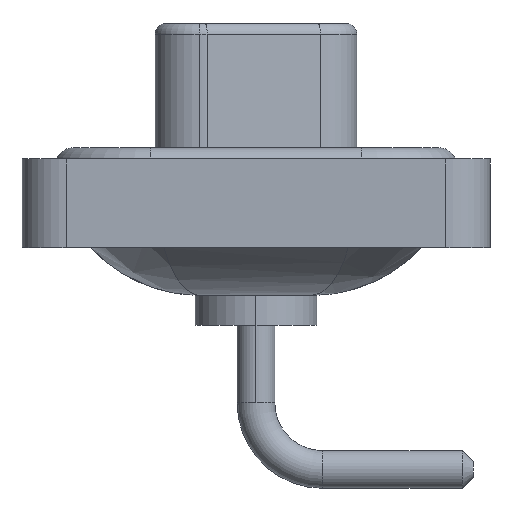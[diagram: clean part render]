
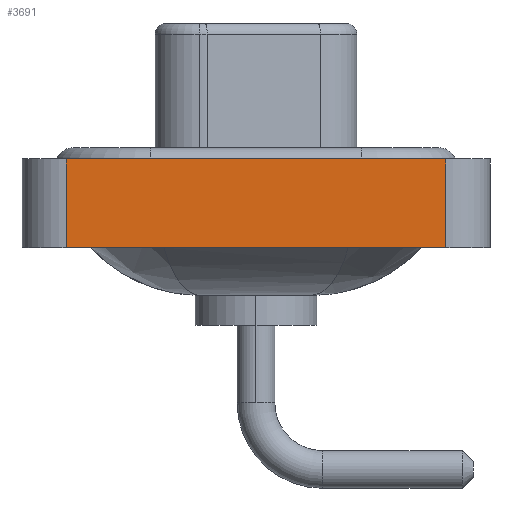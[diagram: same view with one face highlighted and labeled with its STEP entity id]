
A CAD part, left-side view. The second image highlights one B-rep face of the part: STEP entity #3691.
In plain terms, the highlighted planar face has unit normal (-1, 0, 0).
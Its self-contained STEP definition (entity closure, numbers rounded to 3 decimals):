
#387 = EDGE_CURVE ( 'NONE', #12388, #12974, #7501, .T. ) ;
#669 = VERTEX_POINT ( 'NONE', #12848 ) ;
#1430 = ORIENTED_EDGE ( 'NONE', *, *, #1746, .F. ) ;
#1504 = VECTOR ( 'NONE', #5171, 1000. ) ;
#1746 = EDGE_CURVE ( 'NONE', #12974, #669, #2811, .T. ) ;
#2571 = CARTESIAN_POINT ( 'NONE',  ( -7.25, -8.55, -3.6 ) ) ;
#2750 = EDGE_CURVE ( 'NONE', #5761, #669, #7914, .T. ) ;
#2811 = LINE ( 'NONE', #14663, #1504 ) ;
#3085 = LINE ( 'NONE', #9753, #5399 ) ;
#3217 = ORIENTED_EDGE ( 'NONE', *, *, #2750, .T. ) ;
#3414 = PLANE ( 'NONE',  #12436 ) ;
#3490 = DIRECTION ( 'NONE',  ( -1., 0., 0. ) ) ;
#3691 = ADVANCED_FACE ( 'NONE', ( #12682 ), #3414, .T. ) ;
#3801 = EDGE_CURVE ( 'NONE', #12388, #5761, #3085, .T. ) ;
#4676 = ORIENTED_EDGE ( 'NONE', *, *, #387, .F. ) ;
#5171 = DIRECTION ( 'NONE',  ( 0., -1., 0. ) ) ;
#5399 = VECTOR ( 'NONE', #8614, 1000. ) ;
#5761 = VERTEX_POINT ( 'NONE', #2571 ) ;
#7501 = LINE ( 'NONE', #12149, #13327 ) ;
#7914 = LINE ( 'NONE', #12576, #13610 ) ;
#8614 = DIRECTION ( 'NONE',  ( 0., -1., 0. ) ) ;
#8675 = CARTESIAN_POINT ( 'NONE',  ( -7.25, 8.55, 0.4 ) ) ;
#9218 = CARTESIAN_POINT ( 'NONE',  ( -7.25, 8.55, -3.6 ) ) ;
#9753 = CARTESIAN_POINT ( 'NONE',  ( -7.25, -8.55, -3.6 ) ) ;
#11132 = EDGE_LOOP ( 'NONE', ( #3217, #1430, #4676, #13018 ) ) ;
#12149 = CARTESIAN_POINT ( 'NONE',  ( -7.25, 8.55, -3.6 ) ) ;
#12388 = VERTEX_POINT ( 'NONE', #9218 ) ;
#12436 = AXIS2_PLACEMENT_3D ( 'NONE', #12761, #3490, #14962 ) ;
#12499 = DIRECTION ( 'NONE',  ( 0., 0., 1. ) ) ;
#12576 = CARTESIAN_POINT ( 'NONE',  ( -7.25, -8.55, -3.6 ) ) ;
#12682 = FACE_OUTER_BOUND ( 'NONE', #11132, .T. ) ;
#12761 = CARTESIAN_POINT ( 'NONE',  ( -7.25, -8.55, -3.6 ) ) ;
#12848 = CARTESIAN_POINT ( 'NONE',  ( -7.25, -8.55, 0.4 ) ) ;
#12974 = VERTEX_POINT ( 'NONE', #8675 ) ;
#13018 = ORIENTED_EDGE ( 'NONE', *, *, #3801, .T. ) ;
#13327 = VECTOR ( 'NONE', #13524, 1000. ) ;
#13524 = DIRECTION ( 'NONE',  ( 0., 0., 1. ) ) ;
#13610 = VECTOR ( 'NONE', #12499, 1000. ) ;
#14663 = CARTESIAN_POINT ( 'NONE',  ( -7.25, -8.55, 0.4 ) ) ;
#14962 = DIRECTION ( 'NONE',  ( 0., 0., 1. ) ) ;
